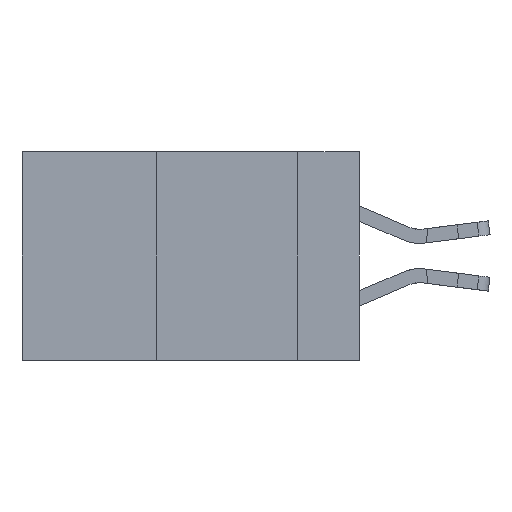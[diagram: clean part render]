
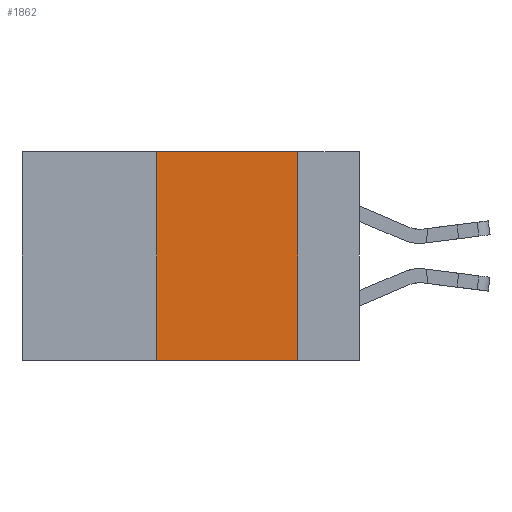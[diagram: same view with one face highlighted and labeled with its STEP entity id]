
A CAD part, left-side view. The second image highlights one B-rep face of the part: STEP entity #1862.
In plain terms, the highlighted planar face has unit normal (-1, 0, 0).
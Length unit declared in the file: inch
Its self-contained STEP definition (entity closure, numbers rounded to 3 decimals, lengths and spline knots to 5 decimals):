
#880 = CARTESIAN_POINT ( 'NONE',  ( 0., 0.6, -0.37 ) ) ;
#931 = EDGE_LOOP ( 'NONE', ( #14508, #15770, #19887, #7816 ) ) ;
#1496 = CARTESIAN_POINT ( 'NONE',  ( 0., 0.6, 0. ) ) ;
#1595 = CARTESIAN_POINT ( 'NONE',  ( 0., 0.11, 0. ) ) ;
#1710 = LINE ( 'NONE', #1595, #9691 ) ;
#1862 = ADVANCED_FACE ( 'NONE', ( #18410 ), #16961, .F. ) ;
#2210 = VERTEX_POINT ( 'NONE', #18231 ) ;
#3608 = VERTEX_POINT ( 'NONE', #7731 ) ;
#3774 = AXIS2_PLACEMENT_3D ( 'NONE', #18921, #17423, #7943 ) ;
#3794 = EDGE_CURVE ( 'NONE', #3608, #2210, #7944, .T. ) ;
#4650 = VECTOR ( 'NONE', #12638, 39.37008 ) ;
#6817 = EDGE_CURVE ( 'NONE', #3608, #19361, #13454, .T. ) ;
#7054 = EDGE_CURVE ( 'NONE', #2210, #11479, #9370, .T. ) ;
#7434 = VECTOR ( 'NONE', #13120, 39.37008 ) ;
#7731 = CARTESIAN_POINT ( 'NONE',  ( 0., 0.36, -0.37 ) ) ;
#7816 = ORIENTED_EDGE ( 'NONE', *, *, #6817, .T. ) ;
#7943 = DIRECTION ( 'NONE',  ( 0., 0., -1. ) ) ;
#7944 = LINE ( 'NONE', #17685, #7434 ) ;
#9370 = LINE ( 'NONE', #1496, #4650 ) ;
#9691 = VECTOR ( 'NONE', #18969, 39.37008 ) ;
#9943 = CARTESIAN_POINT ( 'NONE',  ( 0., 0.11, 0. ) ) ;
#10444 = DIRECTION ( 'NONE',  ( 0., -1., 0. ) ) ;
#11479 = VERTEX_POINT ( 'NONE', #9943 ) ;
#12638 = DIRECTION ( 'NONE',  ( 0., -1., 0. ) ) ;
#13120 = DIRECTION ( 'NONE',  ( 0., 0., 1. ) ) ;
#13454 = LINE ( 'NONE', #880, #17511 ) ;
#14508 = ORIENTED_EDGE ( 'NONE', *, *, #16027, .F. ) ;
#15770 = ORIENTED_EDGE ( 'NONE', *, *, #7054, .F. ) ;
#16027 = EDGE_CURVE ( 'NONE', #11479, #19361, #1710, .T. ) ;
#16576 = CARTESIAN_POINT ( 'NONE',  ( 0., 0.11, -0.37 ) ) ;
#16961 = PLANE ( 'NONE',  #3774 ) ;
#17423 = DIRECTION ( 'NONE',  ( 1., 0., 0. ) ) ;
#17511 = VECTOR ( 'NONE', #10444, 39.37008 ) ;
#17685 = CARTESIAN_POINT ( 'NONE',  ( 0., 0.36, 0. ) ) ;
#18231 = CARTESIAN_POINT ( 'NONE',  ( 0., 0.36, 0. ) ) ;
#18410 = FACE_OUTER_BOUND ( 'NONE', #931, .T. ) ;
#18921 = CARTESIAN_POINT ( 'NONE',  ( 0., 0.6, 0. ) ) ;
#18969 = DIRECTION ( 'NONE',  ( 0., 0., -1. ) ) ;
#19361 = VERTEX_POINT ( 'NONE', #16576 ) ;
#19887 = ORIENTED_EDGE ( 'NONE', *, *, #3794, .F. ) ;
